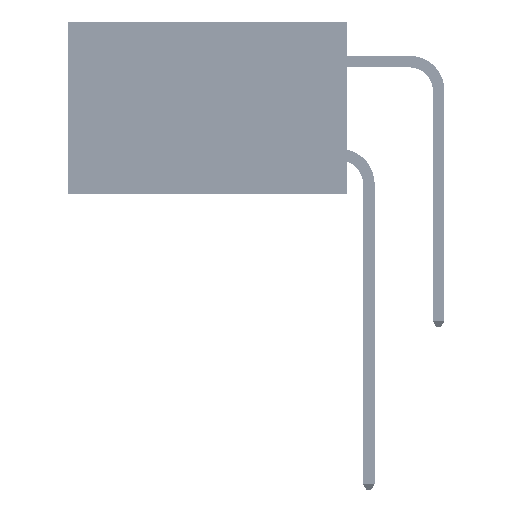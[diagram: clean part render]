
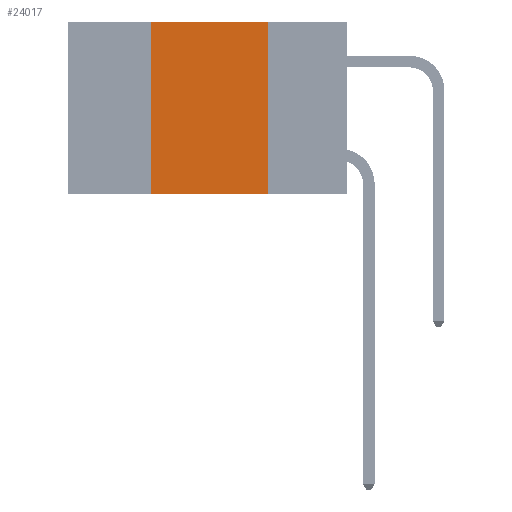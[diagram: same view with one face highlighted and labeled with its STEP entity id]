
A CAD part, left-side view. The second image highlights one B-rep face of the part: STEP entity #24017.
In plain terms, the highlighted planar face has unit normal (-1, 0, 0).
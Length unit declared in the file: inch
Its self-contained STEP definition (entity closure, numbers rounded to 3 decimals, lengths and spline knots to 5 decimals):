
#10 = EDGE_LOOP ( 'NONE', ( #38065, #5659, #9158, #10292 ) ) ;
#1116 = VERTEX_POINT ( 'NONE', #32764 ) ;
#3778 = DIRECTION ( 'NONE',  ( 0., 0., -1. ) ) ;
#5659 = ORIENTED_EDGE ( 'NONE', *, *, #23594, .F. ) ;
#5729 = VERTEX_POINT ( 'NONE', #36258 ) ;
#8280 = LINE ( 'NONE', #34982, #29317 ) ;
#9158 = ORIENTED_EDGE ( 'NONE', *, *, #11810, .F. ) ;
#10292 = ORIENTED_EDGE ( 'NONE', *, *, #44704, .T. ) ;
#11810 = EDGE_CURVE ( 'NONE', #17163, #5729, #12728, .T. ) ;
#12728 = LINE ( 'NONE', #15987, #22710 ) ;
#12856 = CARTESIAN_POINT ( 'NONE',  ( 0., 0.42, -0.37 ) ) ;
#15987 = CARTESIAN_POINT ( 'NONE',  ( 0., 0.42, 0. ) ) ;
#16287 = LINE ( 'NONE', #35066, #25091 ) ;
#16646 = DIRECTION ( 'NONE',  ( 0., -1., 0. ) ) ;
#17163 = VERTEX_POINT ( 'NONE', #12856 ) ;
#20368 = CARTESIAN_POINT ( 'NONE',  ( 0., 0.17, 0. ) ) ;
#22710 = VECTOR ( 'NONE', #38042, 39.37008 ) ;
#23594 = EDGE_CURVE ( 'NONE', #5729, #1116, #8280, .T. ) ;
#24017 = ADVANCED_FACE ( 'NONE', ( #40010 ), #40587, .F. ) ;
#24574 = VERTEX_POINT ( 'NONE', #36181 ) ;
#25091 = VECTOR ( 'NONE', #16646, 39.37008 ) ;
#25730 = AXIS2_PLACEMENT_3D ( 'NONE', #44187, #26202, #3778 ) ;
#26202 = DIRECTION ( 'NONE',  ( 1., 0., 0. ) ) ;
#29317 = VECTOR ( 'NONE', #38584, 39.37008 ) ;
#30417 = LINE ( 'NONE', #20368, #38868 ) ;
#31781 = EDGE_CURVE ( 'NONE', #1116, #24574, #30417, .T. ) ;
#32764 = CARTESIAN_POINT ( 'NONE',  ( 0., 0.17, 0. ) ) ;
#34982 = CARTESIAN_POINT ( 'NONE',  ( 0., 0.6, 0. ) ) ;
#35066 = CARTESIAN_POINT ( 'NONE',  ( 0., 0.6, -0.37 ) ) ;
#36181 = CARTESIAN_POINT ( 'NONE',  ( 0., 0.17, -0.37 ) ) ;
#36258 = CARTESIAN_POINT ( 'NONE',  ( 0., 0.42, 0. ) ) ;
#38042 = DIRECTION ( 'NONE',  ( 0., 0., 1. ) ) ;
#38065 = ORIENTED_EDGE ( 'NONE', *, *, #31781, .F. ) ;
#38584 = DIRECTION ( 'NONE',  ( 0., -1., 0. ) ) ;
#38868 = VECTOR ( 'NONE', #45844, 39.37008 ) ;
#40010 = FACE_OUTER_BOUND ( 'NONE', #10, .T. ) ;
#40587 = PLANE ( 'NONE',  #25730 ) ;
#44187 = CARTESIAN_POINT ( 'NONE',  ( 0., 0.6, 0. ) ) ;
#44704 = EDGE_CURVE ( 'NONE', #17163, #24574, #16287, .T. ) ;
#45844 = DIRECTION ( 'NONE',  ( 0., 0., -1. ) ) ;
